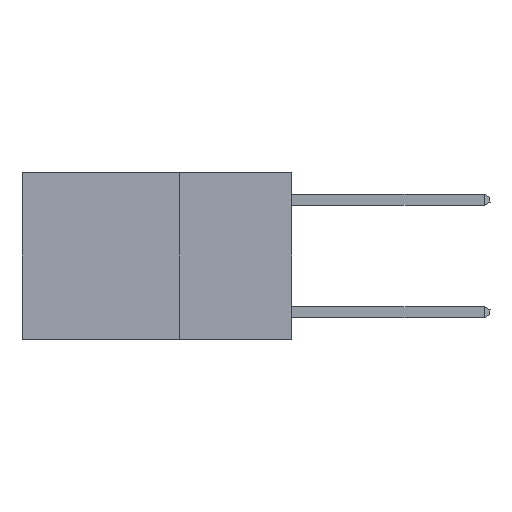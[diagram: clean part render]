
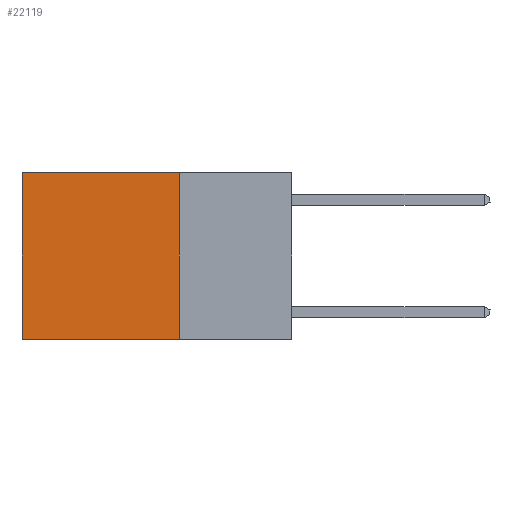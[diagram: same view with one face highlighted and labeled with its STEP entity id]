
A CAD part, left-side view. The second image highlights one B-rep face of the part: STEP entity #22119.
In plain terms, the highlighted planar face has unit normal (-1, 0, 0).
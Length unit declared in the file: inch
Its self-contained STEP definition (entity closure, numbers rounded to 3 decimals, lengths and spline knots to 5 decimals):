
#215 = DIRECTION ( 'NONE',  ( 0., 0., -1. ) ) ;
#1814 = VECTOR ( 'NONE', #24769, 39.37008 ) ;
#1856 = EDGE_CURVE ( 'NONE', #31572, #13722, #20779, .T. ) ;
#2375 = CARTESIAN_POINT ( 'NONE',  ( 0.2625, 0.25, -0.37 ) ) ;
#2575 = LINE ( 'NONE', #10269, #1814 ) ;
#2838 = CARTESIAN_POINT ( 'NONE',  ( 0.2625, 0.25, 0. ) ) ;
#2951 = LINE ( 'NONE', #14929, #28143 ) ;
#4239 = VECTOR ( 'NONE', #5632, 39.37008 ) ;
#4374 = ORIENTED_EDGE ( 'NONE', *, *, #22787, .F. ) ;
#5632 = DIRECTION ( 'NONE',  ( 0., 0., -1. ) ) ;
#7218 = VERTEX_POINT ( 'NONE', #20691 ) ;
#7365 = EDGE_LOOP ( 'NONE', ( #17703, #8126, #4374, #12524 ) ) ;
#8126 = ORIENTED_EDGE ( 'NONE', *, *, #1856, .F. ) ;
#9657 = PLANE ( 'NONE',  #16634 ) ;
#10269 = CARTESIAN_POINT ( 'NONE',  ( 0.2625, 0.25, 0. ) ) ;
#12524 = ORIENTED_EDGE ( 'NONE', *, *, #20026, .T. ) ;
#13722 = VERTEX_POINT ( 'NONE', #28031 ) ;
#14264 = EDGE_CURVE ( 'NONE', #7218, #13722, #23672, .T. ) ;
#14379 = FACE_OUTER_BOUND ( 'NONE', #7365, .T. ) ;
#14644 = CARTESIAN_POINT ( 'NONE',  ( 0.2625, 0.25, 0. ) ) ;
#14783 = CARTESIAN_POINT ( 'NONE',  ( 0.2625, 0.25, -0.37 ) ) ;
#14929 = CARTESIAN_POINT ( 'NONE',  ( 0.2625, 0.25, 0. ) ) ;
#15717 = VERTEX_POINT ( 'NONE', #2838 ) ;
#16634 = AXIS2_PLACEMENT_3D ( 'NONE', #14644, #23439, #17082 ) ;
#17048 = DIRECTION ( 'NONE',  ( 0., 1., 0. ) ) ;
#17082 = DIRECTION ( 'NONE',  ( 0., 0., -1. ) ) ;
#17703 = ORIENTED_EDGE ( 'NONE', *, *, #14264, .T. ) ;
#20026 = EDGE_CURVE ( 'NONE', #15717, #7218, #2575, .T. ) ;
#20691 = CARTESIAN_POINT ( 'NONE',  ( 0.2625, 0.6, 0. ) ) ;
#20779 = LINE ( 'NONE', #2375, #27245 ) ;
#22119 = ADVANCED_FACE ( 'NONE', ( #14379 ), #9657, .F. ) ;
#22667 = CARTESIAN_POINT ( 'NONE',  ( 0.2625, 0.6, 0. ) ) ;
#22787 = EDGE_CURVE ( 'NONE', #15717, #31572, #2951, .T. ) ;
#23439 = DIRECTION ( 'NONE',  ( 1., 0., 0. ) ) ;
#23672 = LINE ( 'NONE', #22667, #4239 ) ;
#24769 = DIRECTION ( 'NONE',  ( 0., 1., 0. ) ) ;
#27245 = VECTOR ( 'NONE', #17048, 39.37008 ) ;
#28031 = CARTESIAN_POINT ( 'NONE',  ( 0.2625, 0.6, -0.37 ) ) ;
#28143 = VECTOR ( 'NONE', #215, 39.37008 ) ;
#31572 = VERTEX_POINT ( 'NONE', #14783 ) ;
